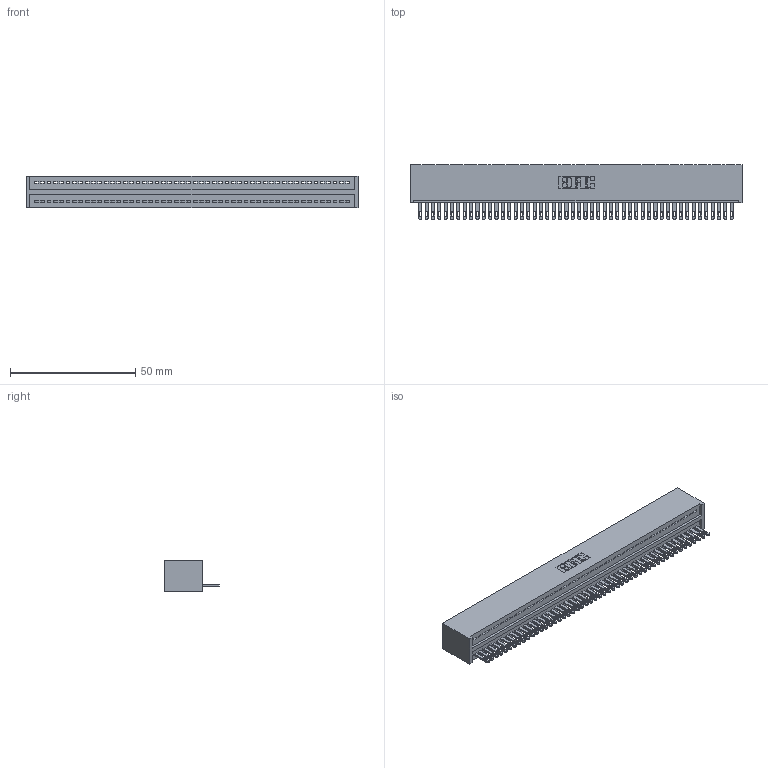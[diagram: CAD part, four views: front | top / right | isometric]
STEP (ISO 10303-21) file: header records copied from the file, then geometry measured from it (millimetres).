
FILE_DESCRIPTION (( 'STEP AP203' ), '1' );
FILE_NAME ('325-050-500-101.STEP', '2020-02-24T23:44:05', ( '' ), ( '' ), 'SwSTEP 2.0', 'SolidWorks 2016', '' );
FILE_SCHEMA (( 'CONFIG_CONTROL_DESIGN' ));
Length unit declared in the file: inch
Products named in the file (3): 325 Part_Lugless; 325-050-500-101; 325-292-001_325-293-100
Assembly tree (51 placements, depth 2):
  325-050-500-101
    325 Part_Lugless
    325-292-001_325-293-100  x50
Bounding box: 132.64 x 21.84 x 12.45 mm (x, y, z)
Volume: 17504.1 mm3; surface area: 19866.4 mm2
Topology: 51 solids, 51 shells, 2806 faces, 8687 edges, 5790 vertices
Faces by surface type: plane 1866, cylinder 940
Entity records: 29185 total; most frequent: CARTESIAN_POINT 5040, ORIENTED_EDGE 5026, DIRECTION 4229, EDGE_CURVE 2513, VECTOR 2389, LINE 2389, VERTEX_POINT 1674, AXIS2_PLACEMENT_3D 920
